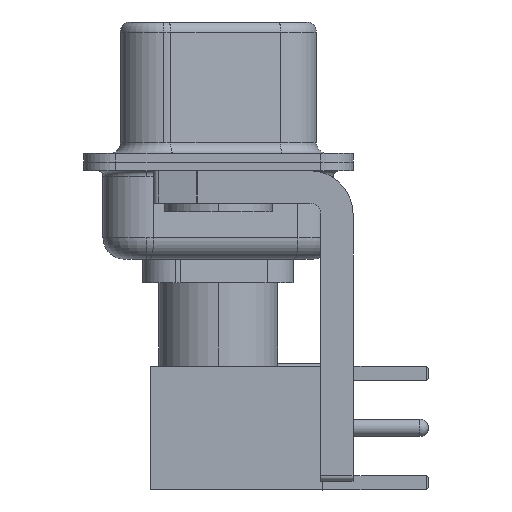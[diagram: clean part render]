
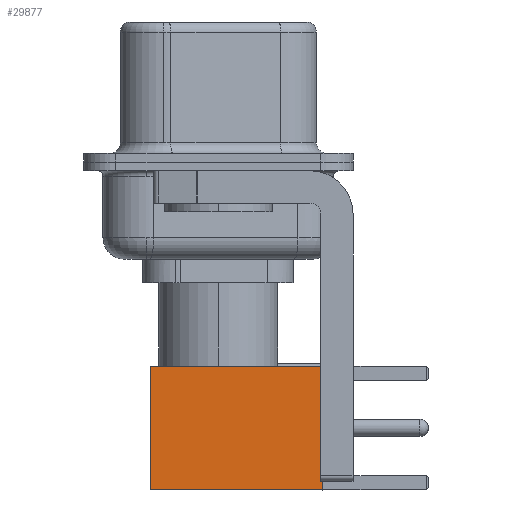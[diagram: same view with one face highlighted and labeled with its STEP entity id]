
A CAD part, left-side view. The second image highlights one B-rep face of the part: STEP entity #29877.
In plain terms, the highlighted face is planar.
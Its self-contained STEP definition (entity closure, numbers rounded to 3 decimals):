
#91 = CARTESIAN_POINT ( 'NONE',  ( 0., 2.875, 8. ) ) ;
#737 = FACE_OUTER_BOUND ( 'NONE', #12671, .T. ) ;
#898 = DIRECTION ( 'NONE',  ( 0., 1., 0. ) ) ;
#2924 = LINE ( 'NONE', #5894, #18419 ) ;
#4349 = VECTOR ( 'NONE', #27176, 1000. ) ;
#4489 = DIRECTION ( 'NONE',  ( -1., 0., 0. ) ) ;
#4778 = AXIS2_PLACEMENT_3D ( 'NONE', #20425, #898, #30950 ) ;
#5087 = VERTEX_POINT ( 'NONE', #24478 ) ;
#5456 = CARTESIAN_POINT ( 'NONE',  ( -2.875, 2.875, 0. ) ) ;
#5722 = DIRECTION ( 'NONE',  ( 0., 0., -1. ) ) ;
#5894 = CARTESIAN_POINT ( 'NONE',  ( -2.875, 2.875, 0. ) ) ;
#6686 = LINE ( 'NONE', #19775, #4349 ) ;
#8495 = ORIENTED_EDGE ( 'NONE', *, *, #31724, .F. ) ;
#9204 = ORIENTED_EDGE ( 'NONE', *, *, #24502, .F. ) ;
#10414 = PLANE ( 'NONE',  #4778 ) ;
#12030 = CARTESIAN_POINT ( 'NONE',  ( 0., 2.875, 0. ) ) ;
#12156 = ORIENTED_EDGE ( 'NONE', *, *, #14184, .T. ) ;
#12671 = EDGE_LOOP ( 'NONE', ( #29008, #12156, #9204, #8495 ) ) ;
#12682 = VERTEX_POINT ( 'NONE', #26356 ) ;
#14184 = EDGE_CURVE ( 'NONE', #12682, #20100, #14660, .T. ) ;
#14660 = LINE ( 'NONE', #12030, #20469 ) ;
#18419 = VECTOR ( 'NONE', #5722, 1000. ) ;
#19775 = CARTESIAN_POINT ( 'NONE',  ( 2.875, 2.875, 0. ) ) ;
#20100 = VERTEX_POINT ( 'NONE', #5456 ) ;
#20260 = DIRECTION ( 'NONE',  ( -1., 0., 0. ) ) ;
#20425 = CARTESIAN_POINT ( 'NONE',  ( 2.875, 2.875, 0. ) ) ;
#20469 = VECTOR ( 'NONE', #4489, 1000. ) ;
#22567 = LINE ( 'NONE', #91, #23191 ) ;
#23191 = VECTOR ( 'NONE', #20260, 1000. ) ;
#24416 = VERTEX_POINT ( 'NONE', #26499 ) ;
#24478 = CARTESIAN_POINT ( 'NONE',  ( 2.875, 2.875, 8. ) ) ;
#24502 = EDGE_CURVE ( 'NONE', #24416, #20100, #2924, .T. ) ;
#26356 = CARTESIAN_POINT ( 'NONE',  ( 2.875, 2.875, 0. ) ) ;
#26499 = CARTESIAN_POINT ( 'NONE',  ( -2.875, 2.875, 8. ) ) ;
#27176 = DIRECTION ( 'NONE',  ( 0., 0., -1. ) ) ;
#29008 = ORIENTED_EDGE ( 'NONE', *, *, #31494, .T. ) ;
#29877 = ADVANCED_FACE ( 'NONE', ( #737 ), #10414, .T. ) ;
#30950 = DIRECTION ( 'NONE',  ( 0., 0., 1. ) ) ;
#31494 = EDGE_CURVE ( 'NONE', #5087, #12682, #6686, .T. ) ;
#31724 = EDGE_CURVE ( 'NONE', #5087, #24416, #22567, .T. ) ;
